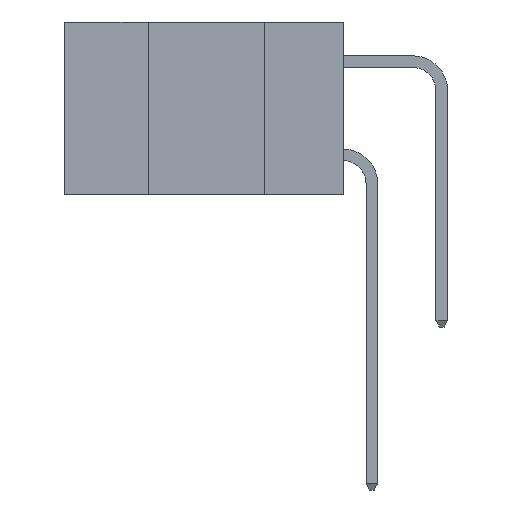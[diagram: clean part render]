
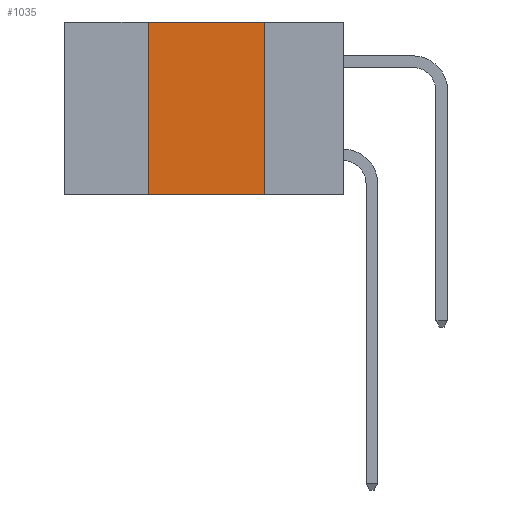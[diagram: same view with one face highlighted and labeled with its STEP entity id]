
A CAD part, left-side view. The second image highlights one B-rep face of the part: STEP entity #1035.
In plain terms, the highlighted planar face has unit normal (-1, 0, 0).
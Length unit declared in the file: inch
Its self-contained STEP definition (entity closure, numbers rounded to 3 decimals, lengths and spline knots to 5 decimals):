
#127 = VERTEX_POINT ( 'NONE', #2097 ) ;
#320 = PLANE ( 'NONE',  #6891 ) ;
#604 = ORIENTED_EDGE ( 'NONE', *, *, #5027, .F. ) ;
#1035 = ADVANCED_FACE ( 'NONE', ( #11961 ), #320, .F. ) ;
#1049 = ORIENTED_EDGE ( 'NONE', *, *, #12448, .F. ) ;
#1237 = VECTOR ( 'NONE', #8999, 39.37008 ) ;
#1565 = CARTESIAN_POINT ( 'NONE',  ( 0., 0.42, -0.37 ) ) ;
#2097 = CARTESIAN_POINT ( 'NONE',  ( 0., 0.42, -0.37 ) ) ;
#2162 = CARTESIAN_POINT ( 'NONE',  ( 0., 0.42, 0. ) ) ;
#2325 = LINE ( 'NONE', #1565, #12309 ) ;
#3509 = CARTESIAN_POINT ( 'NONE',  ( 0., 0.17, 0. ) ) ;
#3901 = EDGE_CURVE ( 'NONE', #127, #5564, #2325, .T. ) ;
#4456 = ORIENTED_EDGE ( 'NONE', *, *, #11912, .T. ) ;
#5027 = EDGE_CURVE ( 'NONE', #5564, #7526, #8916, .T. ) ;
#5564 = VERTEX_POINT ( 'NONE', #2162 ) ;
#5659 = CARTESIAN_POINT ( 'NONE',  ( 0., 0.17, -0.37 ) ) ;
#6034 = DIRECTION ( 'NONE',  ( 0., 0., 1. ) ) ;
#6891 = AXIS2_PLACEMENT_3D ( 'NONE', #11823, #8511, #10227 ) ;
#7147 = VERTEX_POINT ( 'NONE', #7698 ) ;
#7526 = VERTEX_POINT ( 'NONE', #3509 ) ;
#7532 = LINE ( 'NONE', #5659, #9859 ) ;
#7607 = CARTESIAN_POINT ( 'NONE',  ( 0., 0.6, -0.37 ) ) ;
#7698 = CARTESIAN_POINT ( 'NONE',  ( 0., 0.17, -0.37 ) ) ;
#7913 = ORIENTED_EDGE ( 'NONE', *, *, #3901, .F. ) ;
#8003 = CARTESIAN_POINT ( 'NONE',  ( 0., 0.6, 0. ) ) ;
#8511 = DIRECTION ( 'NONE',  ( 1., 0., 0. ) ) ;
#8916 = LINE ( 'NONE', #8003, #1237 ) ;
#8999 = DIRECTION ( 'NONE',  ( 0., -1., 0. ) ) ;
#9859 = VECTOR ( 'NONE', #11539, 39.37008 ) ;
#10227 = DIRECTION ( 'NONE',  ( 0., 0., -1. ) ) ;
#10389 = EDGE_LOOP ( 'NONE', ( #1049, #604, #7913, #4456 ) ) ;
#11088 = VECTOR ( 'NONE', #11512, 39.37008 ) ;
#11512 = DIRECTION ( 'NONE',  ( 0., -1., 0. ) ) ;
#11539 = DIRECTION ( 'NONE',  ( 0., 0., -1. ) ) ;
#11708 = LINE ( 'NONE', #7607, #11088 ) ;
#11823 = CARTESIAN_POINT ( 'NONE',  ( 0., 0.6, 0. ) ) ;
#11912 = EDGE_CURVE ( 'NONE', #127, #7147, #11708, .T. ) ;
#11961 = FACE_OUTER_BOUND ( 'NONE', #10389, .T. ) ;
#12309 = VECTOR ( 'NONE', #6034, 39.37008 ) ;
#12448 = EDGE_CURVE ( 'NONE', #7526, #7147, #7532, .T. ) ;
